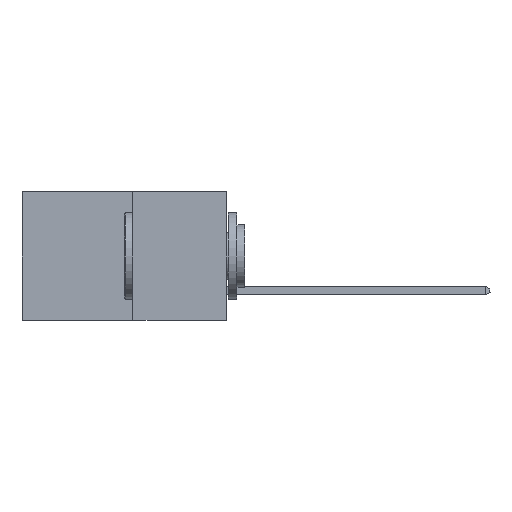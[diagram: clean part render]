
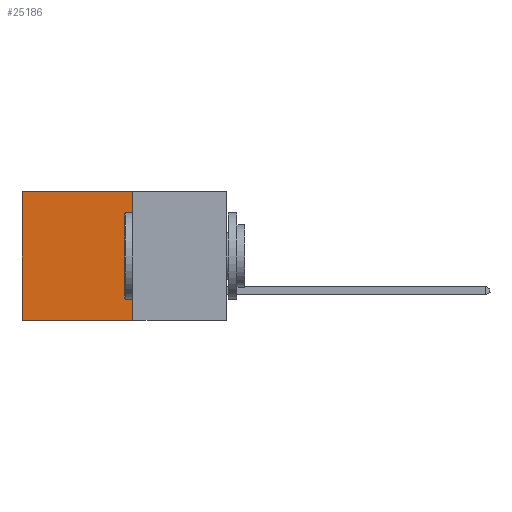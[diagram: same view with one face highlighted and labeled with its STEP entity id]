
A CAD part, left-side view. The second image highlights one B-rep face of the part: STEP entity #25186.
In plain terms, the highlighted planar face has unit normal (-1, 0, 0).
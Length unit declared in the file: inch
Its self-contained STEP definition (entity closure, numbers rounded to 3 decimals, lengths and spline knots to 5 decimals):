
#102 = EDGE_CURVE ( 'NONE', #26381, #6239, #6528, .T. ) ;
#821 = CARTESIAN_POINT ( 'NONE',  ( 0.277, 0.27, 0. ) ) ;
#3783 = DIRECTION ( 'NONE',  ( 1., 0., 0. ) ) ;
#4284 = ORIENTED_EDGE ( 'NONE', *, *, #26852, .F. ) ;
#5806 = CARTESIAN_POINT ( 'NONE',  ( 0.277, 0.27, -0.37 ) ) ;
#6239 = VERTEX_POINT ( 'NONE', #24745 ) ;
#6528 = LINE ( 'NONE', #19139, #18110 ) ;
#7571 = ORIENTED_EDGE ( 'NONE', *, *, #102, .T. ) ;
#7853 = VECTOR ( 'NONE', #16473, 39.37008 ) ;
#8089 = VERTEX_POINT ( 'NONE', #5806 ) ;
#9174 = EDGE_CURVE ( 'NONE', #8089, #15107, #19974, .T. ) ;
#10870 = AXIS2_PLACEMENT_3D ( 'NONE', #24578, #3783, #19999 ) ;
#12844 = DIRECTION ( 'NONE',  ( 0., 1., 0. ) ) ;
#13997 = LINE ( 'NONE', #28008, #7853 ) ;
#15107 = VERTEX_POINT ( 'NONE', #19060 ) ;
#15352 = ORIENTED_EDGE ( 'NONE', *, *, #29956, .T. ) ;
#15361 = PLANE ( 'NONE',  #10870 ) ;
#16473 = DIRECTION ( 'NONE',  ( 0., 0., -1. ) ) ;
#17002 = CARTESIAN_POINT ( 'NONE',  ( 0.277, 0.59, -0.37 ) ) ;
#18110 = VECTOR ( 'NONE', #23391, 39.37008 ) ;
#18810 = FACE_OUTER_BOUND ( 'NONE', #26459, .T. ) ;
#19060 = CARTESIAN_POINT ( 'NONE',  ( 0.277, 0.59, -0.37 ) ) ;
#19139 = CARTESIAN_POINT ( 'NONE',  ( 0.277, 0.27, 0. ) ) ;
#19316 = DIRECTION ( 'NONE',  ( 0., 0., -1. ) ) ;
#19974 = LINE ( 'NONE', #22048, #24698 ) ;
#19999 = DIRECTION ( 'NONE',  ( 0., 0., -1. ) ) ;
#22048 = CARTESIAN_POINT ( 'NONE',  ( 0.277, 0.27, -0.37 ) ) ;
#23391 = DIRECTION ( 'NONE',  ( 0., 1., 0. ) ) ;
#24578 = CARTESIAN_POINT ( 'NONE',  ( 0.277, 0.27, -0.37 ) ) ;
#24698 = VECTOR ( 'NONE', #12844, 39.37008 ) ;
#24710 = VECTOR ( 'NONE', #19316, 39.37008 ) ;
#24745 = CARTESIAN_POINT ( 'NONE',  ( 0.277, 0.59, 0. ) ) ;
#25186 = ADVANCED_FACE ( 'NONE', ( #18810 ), #15361, .F. ) ;
#25421 = LINE ( 'NONE', #17002, #24710 ) ;
#25982 = ORIENTED_EDGE ( 'NONE', *, *, #9174, .F. ) ;
#26381 = VERTEX_POINT ( 'NONE', #821 ) ;
#26459 = EDGE_LOOP ( 'NONE', ( #15352, #25982, #4284, #7571 ) ) ;
#26852 = EDGE_CURVE ( 'NONE', #26381, #8089, #13997, .T. ) ;
#28008 = CARTESIAN_POINT ( 'NONE',  ( 0.277, 0.27, -0.37 ) ) ;
#29956 = EDGE_CURVE ( 'NONE', #6239, #15107, #25421, .T. ) ;
